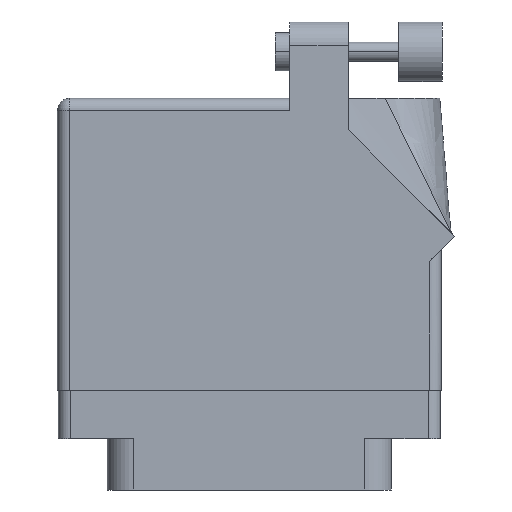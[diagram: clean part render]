
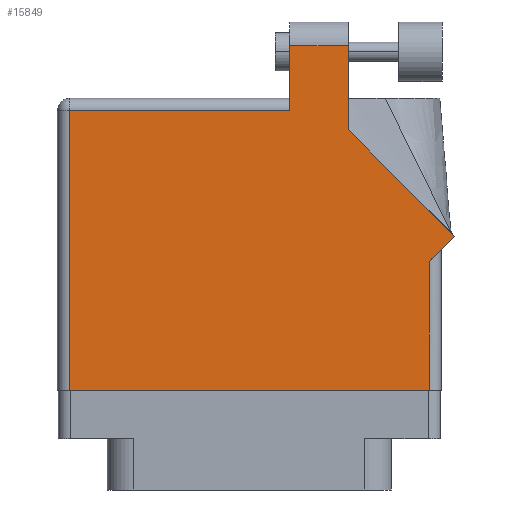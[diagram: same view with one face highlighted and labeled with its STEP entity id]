
A CAD part, front view. The second image highlights one B-rep face of the part: STEP entity #15849.
In plain terms, the highlighted face is planar.
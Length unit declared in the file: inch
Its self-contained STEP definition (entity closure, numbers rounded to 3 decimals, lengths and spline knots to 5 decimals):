
#1282 = CARTESIAN_POINT ( 'NONE',  ( 0.212, 1.43, 0.455 ) ) ;
#1351 = EDGE_LOOP ( 'NONE', ( #38979, #22265, #31925, #7856, #24692, #29623, #20277, #9101, #25889 ) ) ;
#2460 = VERTEX_POINT ( 'NONE', #6510 ) ;
#3264 = CARTESIAN_POINT ( 'NONE',  ( 0.212, 1.705, 0.455 ) ) ;
#3499 = EDGE_CURVE ( 'NONE', #34546, #22006, #26234, .T. ) ;
#4136 = CARTESIAN_POINT ( 'NONE',  ( 0.519, 1.26442, 0.455 ) ) ;
#4468 = LINE ( 'NONE', #1282, #4960 ) ;
#4960 = VECTOR ( 'NONE', #32534, 39.37008 ) ;
#5326 = DIRECTION ( 'NONE',  ( -0.707, 0.707, 0. ) ) ;
#5695 = LINE ( 'NONE', #14981, #34446 ) ;
#5883 = CARTESIAN_POINT ( 'NONE',  ( -1.005, 1.43, 0.455 ) ) ;
#6176 = CARTESIAN_POINT ( 'NONE',  ( 0.943, -0.1, 0.455 ) ) ;
#6510 = CARTESIAN_POINT ( 'NONE',  ( 0.212, 1.368, 0.455 ) ) ;
#7697 = VECTOR ( 'NONE', #19381, 39.37008 ) ;
#7856 = ORIENTED_EDGE ( 'NONE', *, *, #13297, .T. ) ;
#8987 = EDGE_CURVE ( 'NONE', #28126, #34546, #32067, .T. ) ;
#9101 = ORIENTED_EDGE ( 'NONE', *, *, #23501, .T. ) ;
#9851 = VECTOR ( 'NONE', #13669, 39.37008 ) ;
#10142 = CARTESIAN_POINT ( 'NONE',  ( -0.943, 1.368, 0.455 ) ) ;
#11364 = FACE_OUTER_BOUND ( 'NONE', #1351, .T. ) ;
#12143 = VERTEX_POINT ( 'NONE', #10142 ) ;
#12164 = DIRECTION ( 'NONE',  ( -1., 0., 0. ) ) ;
#12309 = AXIS2_PLACEMENT_3D ( 'NONE', #5883, #30800, #12164 ) ;
#12315 = EDGE_CURVE ( 'NONE', #33395, #22806, #16203, .T. ) ;
#12493 = DIRECTION ( 'NONE',  ( 0.707, 0.707, 0. ) ) ;
#12794 = CARTESIAN_POINT ( 'NONE',  ( 1.07571, 0.70771, 0.455 ) ) ;
#13297 = EDGE_CURVE ( 'NONE', #2460, #12143, #23737, .T. ) ;
#13669 = DIRECTION ( 'NONE',  ( 0., 1., 0. ) ) ;
#14981 = CARTESIAN_POINT ( 'NONE',  ( 0.212, 1.705, 0.455 ) ) ;
#15607 = VERTEX_POINT ( 'NONE', #38915 ) ;
#15849 = ADVANCED_FACE ( 'NONE', ( #11364 ), #24544, .F. ) ;
#16203 = LINE ( 'NONE', #30518, #30811 ) ;
#17923 = CARTESIAN_POINT ( 'NONE',  ( -0.943, -0.1, 0.455 ) ) ;
#19381 = DIRECTION ( 'NONE',  ( 1., 0., 0. ) ) ;
#20068 = LINE ( 'NONE', #4136, #9851 ) ;
#20277 = ORIENTED_EDGE ( 'NONE', *, *, #3499, .T. ) ;
#21646 = DIRECTION ( 'NONE',  ( -1., 0., 0. ) ) ;
#22006 = VERTEX_POINT ( 'NONE', #22463 ) ;
#22265 = ORIENTED_EDGE ( 'NONE', *, *, #40019, .T. ) ;
#22421 = DIRECTION ( 'NONE',  ( 0., 1., 0. ) ) ;
#22463 = CARTESIAN_POINT ( 'NONE',  ( 0.943, 0.575, 0.455 ) ) ;
#22476 = LINE ( 'NONE', #24724, #23900 ) ;
#22806 = VERTEX_POINT ( 'NONE', #27363 ) ;
#23501 = EDGE_CURVE ( 'NONE', #22006, #33395, #22476, .T. ) ;
#23737 = LINE ( 'NONE', #37181, #25708 ) ;
#23900 = VECTOR ( 'NONE', #12493, 39.37008 ) ;
#24544 = PLANE ( 'NONE',  #12309 ) ;
#24692 = ORIENTED_EDGE ( 'NONE', *, *, #36227, .T. ) ;
#24724 = CARTESIAN_POINT ( 'NONE',  ( 1.005, 0.637, 0.455 ) ) ;
#24761 = DIRECTION ( 'NONE',  ( -1., 0., 0. ) ) ;
#25139 = CARTESIAN_POINT ( 'NONE',  ( 0.943, 0.637, 0.455 ) ) ;
#25708 = VECTOR ( 'NONE', #21646, 39.37008 ) ;
#25889 = ORIENTED_EDGE ( 'NONE', *, *, #12315, .T. ) ;
#26234 = LINE ( 'NONE', #25139, #33518 ) ;
#26885 = DIRECTION ( 'NONE',  ( 0., -1., 0. ) ) ;
#27363 = CARTESIAN_POINT ( 'NONE',  ( 0.519, 1.26442, 0.455 ) ) ;
#27870 = VECTOR ( 'NONE', #26885, 39.37008 ) ;
#28126 = VERTEX_POINT ( 'NONE', #38720 ) ;
#29623 = ORIENTED_EDGE ( 'NONE', *, *, #8987, .T. ) ;
#30518 = CARTESIAN_POINT ( 'NONE',  ( 1.07571, 0.70771, 0.455 ) ) ;
#30800 = DIRECTION ( 'NONE',  ( 0., 0., -1. ) ) ;
#30811 = VECTOR ( 'NONE', #5326, 39.37008 ) ;
#30980 = EDGE_CURVE ( 'NONE', #33311, #2460, #4468, .T. ) ;
#31925 = ORIENTED_EDGE ( 'NONE', *, *, #30980, .T. ) ;
#32067 = LINE ( 'NONE', #38016, #7697 ) ;
#32534 = DIRECTION ( 'NONE',  ( 0., -1., 0. ) ) ;
#33311 = VERTEX_POINT ( 'NONE', #3264 ) ;
#33395 = VERTEX_POINT ( 'NONE', #12794 ) ;
#33518 = VECTOR ( 'NONE', #22421, 39.37008 ) ;
#34446 = VECTOR ( 'NONE', #24761, 39.37008 ) ;
#34546 = VERTEX_POINT ( 'NONE', #6176 ) ;
#36171 = LINE ( 'NONE', #17923, #27870 ) ;
#36227 = EDGE_CURVE ( 'NONE', #12143, #28126, #36171, .T. ) ;
#36535 = EDGE_CURVE ( 'NONE', #22806, #15607, #20068, .T. ) ;
#37181 = CARTESIAN_POINT ( 'NONE',  ( -1.005, 1.368, 0.455 ) ) ;
#38016 = CARTESIAN_POINT ( 'NONE',  ( -1.005, -0.1, 0.455 ) ) ;
#38720 = CARTESIAN_POINT ( 'NONE',  ( -0.943, -0.1, 0.455 ) ) ;
#38915 = CARTESIAN_POINT ( 'NONE',  ( 0.519, 1.705, 0.455 ) ) ;
#38979 = ORIENTED_EDGE ( 'NONE', *, *, #36535, .T. ) ;
#40019 = EDGE_CURVE ( 'NONE', #15607, #33311, #5695, .T. ) ;
